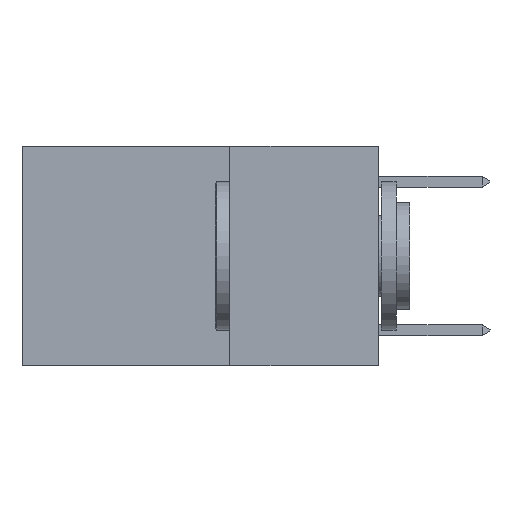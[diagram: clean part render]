
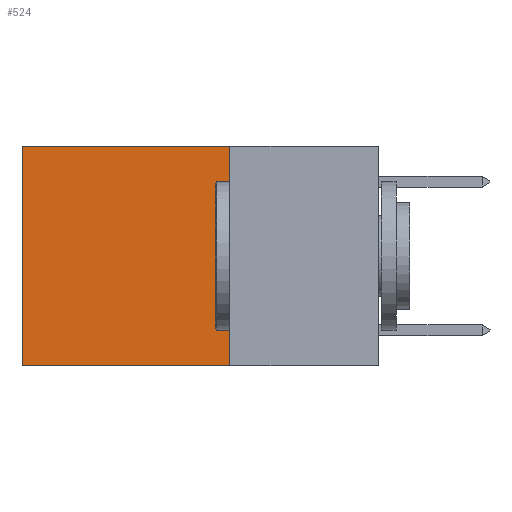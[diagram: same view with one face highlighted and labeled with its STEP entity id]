
A CAD part, left-side view. The second image highlights one B-rep face of the part: STEP entity #524.
In plain terms, the highlighted planar face has unit normal (-1, 0, 0).
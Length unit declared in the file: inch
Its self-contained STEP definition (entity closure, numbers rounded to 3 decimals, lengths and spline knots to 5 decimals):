
#462 = LINE ( 'NONE', #25867, #17454 ) ;
#524 = ADVANCED_FACE ( 'NONE', ( #26942 ), #6187, .F. ) ;
#615 = EDGE_CURVE ( 'NONE', #29113, #22799, #3839, .T. ) ;
#1544 = VECTOR ( 'NONE', #26077, 39.37008 ) ;
#2262 = VECTOR ( 'NONE', #18092, 39.37008 ) ;
#3839 = LINE ( 'NONE', #9444, #17433 ) ;
#4165 = CARTESIAN_POINT ( 'NONE',  ( 0.2625, 0.25, 0. ) ) ;
#4166 = DIRECTION ( 'NONE',  ( 0., 1., 0. ) ) ;
#4931 = CARTESIAN_POINT ( 'NONE',  ( 0.2625, 0.25, 0. ) ) ;
#6187 = PLANE ( 'NONE',  #18568 ) ;
#6725 = CARTESIAN_POINT ( 'NONE',  ( 0.2625, 0.6, 0. ) ) ;
#7015 = ORIENTED_EDGE ( 'NONE', *, *, #615, .F. ) ;
#8052 = CARTESIAN_POINT ( 'NONE',  ( 0.2625, 0.6, -0.37 ) ) ;
#8884 = EDGE_CURVE ( 'NONE', #29113, #17737, #26920, .T. ) ;
#9444 = CARTESIAN_POINT ( 'NONE',  ( 0.2625, 0.25, 0. ) ) ;
#9458 = LINE ( 'NONE', #13465, #2262 ) ;
#11596 = DIRECTION ( 'NONE',  ( 0., 0., -1. ) ) ;
#13465 = CARTESIAN_POINT ( 'NONE',  ( 0.2625, 0.6, 0. ) ) ;
#17433 = VECTOR ( 'NONE', #11596, 39.37008 ) ;
#17454 = VECTOR ( 'NONE', #4166, 39.37008 ) ;
#17737 = VERTEX_POINT ( 'NONE', #6725 ) ;
#18092 = DIRECTION ( 'NONE',  ( 0., 0., -1. ) ) ;
#18182 = EDGE_CURVE ( 'NONE', #17737, #24610, #9458, .T. ) ;
#18568 = AXIS2_PLACEMENT_3D ( 'NONE', #4165, #23519, #21062 ) ;
#19355 = ORIENTED_EDGE ( 'NONE', *, *, #8884, .T. ) ;
#20359 = CARTESIAN_POINT ( 'NONE',  ( 0.2625, 0.25, 0. ) ) ;
#21062 = DIRECTION ( 'NONE',  ( 0., 0., -1. ) ) ;
#22799 = VERTEX_POINT ( 'NONE', #23594 ) ;
#23082 = EDGE_LOOP ( 'NONE', ( #28114, #31263, #7015, #19355 ) ) ;
#23519 = DIRECTION ( 'NONE',  ( 1., 0., 0. ) ) ;
#23594 = CARTESIAN_POINT ( 'NONE',  ( 0.2625, 0.25, -0.37 ) ) ;
#24610 = VERTEX_POINT ( 'NONE', #8052 ) ;
#24706 = EDGE_CURVE ( 'NONE', #22799, #24610, #462, .T. ) ;
#25867 = CARTESIAN_POINT ( 'NONE',  ( 0.2625, 0.25, -0.37 ) ) ;
#26077 = DIRECTION ( 'NONE',  ( 0., 1., 0. ) ) ;
#26920 = LINE ( 'NONE', #20359, #1544 ) ;
#26942 = FACE_OUTER_BOUND ( 'NONE', #23082, .T. ) ;
#28114 = ORIENTED_EDGE ( 'NONE', *, *, #18182, .T. ) ;
#29113 = VERTEX_POINT ( 'NONE', #4931 ) ;
#31263 = ORIENTED_EDGE ( 'NONE', *, *, #24706, .F. ) ;
